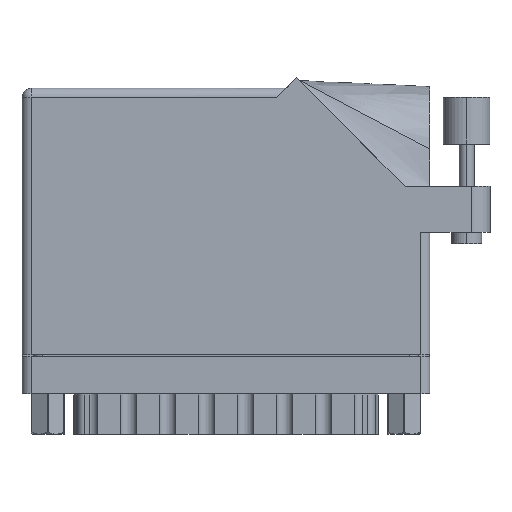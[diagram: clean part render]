
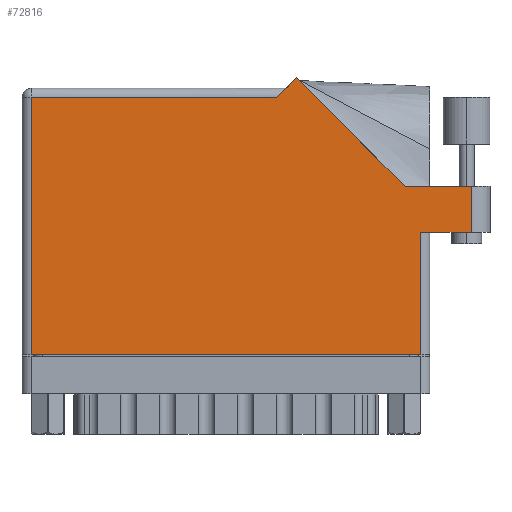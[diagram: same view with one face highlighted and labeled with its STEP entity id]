
A CAD part, front view. The second image highlights one B-rep face of the part: STEP entity #72816.
In plain terms, the highlighted face is planar.
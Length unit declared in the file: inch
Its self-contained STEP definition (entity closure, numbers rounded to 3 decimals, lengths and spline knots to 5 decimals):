
#4457 = CARTESIAN_POINT ( 'NONE',  ( 1.82871, 1.84571, 0. ) ) ;
#4816 = DIRECTION ( 'NONE',  ( 1., 0., 0. ) ) ;
#5116 = DIRECTION ( 'NONE',  ( 0., 1., 0. ) ) ;
#6552 = LINE ( 'NONE', #35430, #54250 ) ;
#7896 = LINE ( 'NONE', #50285, #32262 ) ;
#9628 = CARTESIAN_POINT ( 'NONE',  ( 0.062, 1.713, 0. ) ) ;
#9780 = CARTESIAN_POINT ( 'NONE',  ( 2.55242, 1.122, 0. ) ) ;
#9940 = DIRECTION ( 'NONE',  ( -0.707, -0.707, 0. ) ) ;
#11383 = CARTESIAN_POINT ( 'NONE',  ( 0.062, 0., 0. ) ) ;
#12484 = VECTOR ( 'NONE', #4816, 39.37008 ) ;
#13090 = EDGE_CURVE ( 'NONE', #24848, #55789, #65997, .T. ) ;
#13695 = ORIENTED_EDGE ( 'NONE', *, *, #32659, .T. ) ;
#14022 = ORIENTED_EDGE ( 'NONE', *, *, #34293, .T. ) ;
#14526 = CARTESIAN_POINT ( 'NONE',  ( 1.696, 1.713, 0. ) ) ;
#17224 = ORIENTED_EDGE ( 'NONE', *, *, #26079, .T. ) ;
#17429 = VERTEX_POINT ( 'NONE', #80255 ) ;
#18200 = CARTESIAN_POINT ( 'NONE',  ( 2.656, 0.815, 0. ) ) ;
#18281 = DIRECTION ( 'NONE',  ( -1., 0., 0. ) ) ;
#20771 = DIRECTION ( 'NONE',  ( 0., 1., 0. ) ) ;
#21289 = VERTEX_POINT ( 'NONE', #4457 ) ;
#23145 = ORIENTED_EDGE ( 'NONE', *, *, #13090, .T. ) ;
#24154 = LINE ( 'NONE', #9780, #73728 ) ;
#24848 = VERTEX_POINT ( 'NONE', #11383 ) ;
#25803 = DIRECTION ( 'NONE',  ( -1., 0., 0. ) ) ;
#26079 = EDGE_CURVE ( 'NONE', #55789, #17429, #61710, .T. ) ;
#26081 = CARTESIAN_POINT ( 'NONE',  ( 0., 1.775, 0. ) ) ;
#27510 = CARTESIAN_POINT ( 'NONE',  ( 0.062, 0., 0. ) ) ;
#27749 = EDGE_CURVE ( 'NONE', #37042, #28664, #7896, .T. ) ;
#28664 = VERTEX_POINT ( 'NONE', #9628 ) ;
#29140 = ORIENTED_EDGE ( 'NONE', *, *, #27749, .T. ) ;
#31991 = EDGE_CURVE ( 'NONE', #67932, #59982, #66114, .T. ) ;
#32262 = VECTOR ( 'NONE', #49210, 39.37008 ) ;
#32659 = EDGE_CURVE ( 'NONE', #54292, #21289, #24154, .T. ) ;
#34293 = EDGE_CURVE ( 'NONE', #21289, #37042, #76325, .T. ) ;
#35430 = CARTESIAN_POINT ( 'NONE',  ( 3.118, 1.122, 0. ) ) ;
#36442 = VECTOR ( 'NONE', #5116, 39.37008 ) ;
#37042 = VERTEX_POINT ( 'NONE', #14526 ) ;
#39198 = CARTESIAN_POINT ( 'NONE',  ( 2.993, 1.122, 0. ) ) ;
#40392 = CARTESIAN_POINT ( 'NONE',  ( 1.758, 1.775, 0. ) ) ;
#41101 = EDGE_LOOP ( 'NONE', ( #57876, #62460, #66194, #13695, #14022, #29140, #46246, #23145, #17224 ) ) ;
#42101 = CARTESIAN_POINT ( 'NONE',  ( 0., 0., 0. ) ) ;
#43380 = VECTOR ( 'NONE', #77151, 39.37008 ) ;
#44537 = LINE ( 'NONE', #69239, #49371 ) ;
#46246 = ORIENTED_EDGE ( 'NONE', *, *, #72691, .T. ) ;
#46327 = CARTESIAN_POINT ( 'NONE',  ( 2.993, 0.815, 0. ) ) ;
#46339 = FACE_OUTER_BOUND ( 'NONE', #41101, .T. ) ;
#46998 = AXIS2_PLACEMENT_3D ( 'NONE', #26081, #74976, #25803 ) ;
#47221 = VECTOR ( 'NONE', #9940, 39.37008 ) ;
#49210 = DIRECTION ( 'NONE',  ( -1., 0., 0. ) ) ;
#49371 = VECTOR ( 'NONE', #56757, 39.37008 ) ;
#50285 = CARTESIAN_POINT ( 'NONE',  ( 0., 1.713, 0. ) ) ;
#51070 = PLANE ( 'NONE',  #46998 ) ;
#53266 = DIRECTION ( 'NONE',  ( -0.707, 0.707, 0. ) ) ;
#54250 = VECTOR ( 'NONE', #18281, 39.37008 ) ;
#54292 = VERTEX_POINT ( 'NONE', #78653 ) ;
#55789 = VERTEX_POINT ( 'NONE', #56409 ) ;
#56409 = CARTESIAN_POINT ( 'NONE',  ( 2.656, 0., 0. ) ) ;
#56757 = DIRECTION ( 'NONE',  ( 1., 0., 0. ) ) ;
#57037 = EDGE_CURVE ( 'NONE', #17429, #67932, #44537, .T. ) ;
#57876 = ORIENTED_EDGE ( 'NONE', *, *, #57037, .T. ) ;
#59914 = LINE ( 'NONE', #27510, #43380 ) ;
#59982 = VERTEX_POINT ( 'NONE', #39198 ) ;
#61710 = LINE ( 'NONE', #18200, #36442 ) ;
#62460 = ORIENTED_EDGE ( 'NONE', *, *, #31991, .T. ) ;
#65070 = CARTESIAN_POINT ( 'NONE',  ( 2.993, 1.122, 0. ) ) ;
#65997 = LINE ( 'NONE', #42101, #12484 ) ;
#66114 = LINE ( 'NONE', #65070, #76707 ) ;
#66194 = ORIENTED_EDGE ( 'NONE', *, *, #66837, .T. ) ;
#66837 = EDGE_CURVE ( 'NONE', #59982, #54292, #6552, .T. ) ;
#67932 = VERTEX_POINT ( 'NONE', #46327 ) ;
#69239 = CARTESIAN_POINT ( 'NONE',  ( 2.718, 0.815, 0. ) ) ;
#72691 = EDGE_CURVE ( 'NONE', #28664, #24848, #59914, .T. ) ;
#72816 = ADVANCED_FACE ( 'NONE', ( #46339 ), #51070, .F. ) ;
#73728 = VECTOR ( 'NONE', #53266, 39.37008 ) ;
#74976 = DIRECTION ( 'NONE',  ( 0., 0., -1. ) ) ;
#76325 = LINE ( 'NONE', #40392, #47221 ) ;
#76707 = VECTOR ( 'NONE', #20771, 39.37008 ) ;
#77151 = DIRECTION ( 'NONE',  ( 0., -1., 0. ) ) ;
#78653 = CARTESIAN_POINT ( 'NONE',  ( 2.55242, 1.122, 0. ) ) ;
#80255 = CARTESIAN_POINT ( 'NONE',  ( 2.656, 0.815, 0. ) ) ;
